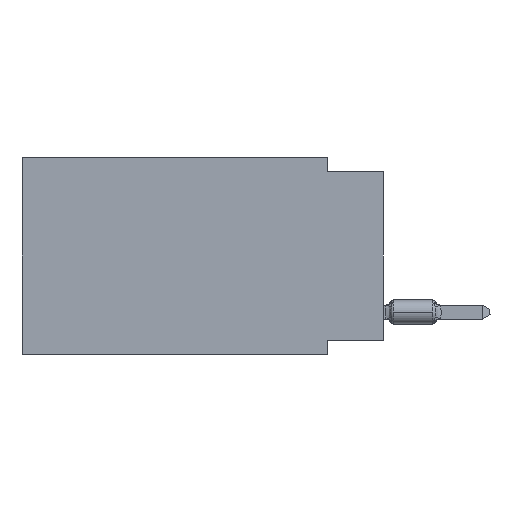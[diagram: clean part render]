
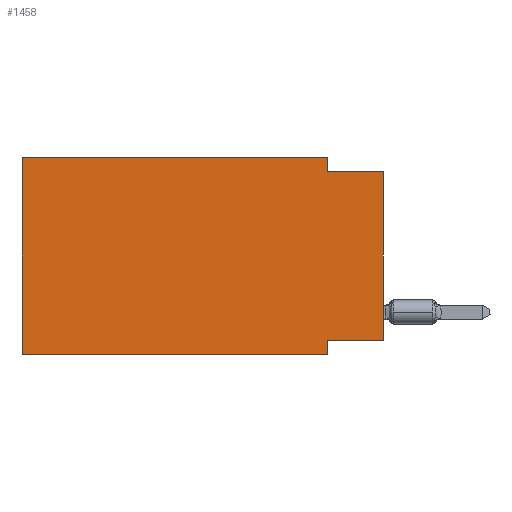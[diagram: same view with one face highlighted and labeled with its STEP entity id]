
A CAD part, left-side view. The second image highlights one B-rep face of the part: STEP entity #1458.
In plain terms, the highlighted planar face has unit normal (-1, 0, 0).
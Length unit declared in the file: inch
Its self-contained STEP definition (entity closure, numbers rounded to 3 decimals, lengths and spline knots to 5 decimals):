
#38 = VERTEX_POINT ( 'NONE', #5850 ) ;
#789 = DIRECTION ( 'NONE',  ( 1., 0., 0. ) ) ;
#1031 = LINE ( 'NONE', #18066, #4574 ) ;
#1359 = CARTESIAN_POINT ( 'NONE',  ( 0., 0., 0. ) ) ;
#1458 = ADVANCED_FACE ( 'NONE', ( #35137 ), #30677, .F. ) ;
#2916 = ORIENTED_EDGE ( 'NONE', *, *, #30691, .F. ) ;
#3138 = CARTESIAN_POINT ( 'NONE',  ( 0., 0.645, 0. ) ) ;
#4574 = VECTOR ( 'NONE', #35098, 39.37008 ) ;
#4625 = VERTEX_POINT ( 'NONE', #49537 ) ;
#5850 = CARTESIAN_POINT ( 'NONE',  ( 0., 0.1, 0. ) ) ;
#7056 = EDGE_CURVE ( 'NONE', #47800, #4625, #20248, .T. ) ;
#7983 = VECTOR ( 'NONE', #36603, 39.37008 ) ;
#9084 = CARTESIAN_POINT ( 'NONE',  ( 0., 0.1, -0.025 ) ) ;
#9440 = LINE ( 'NONE', #1359, #35969 ) ;
#10559 = DIRECTION ( 'NONE',  ( 0., 0., -1. ) ) ;
#11693 = DIRECTION ( 'NONE',  ( 0., 0., -1. ) ) ;
#12225 = EDGE_CURVE ( 'NONE', #38, #33472, #21179, .T. ) ;
#12871 = CARTESIAN_POINT ( 'NONE',  ( 0., 0., -0.025 ) ) ;
#13018 = CARTESIAN_POINT ( 'NONE',  ( 0., 0.645, -0.35 ) ) ;
#14031 = CARTESIAN_POINT ( 'NONE',  ( 0., 0.1, -0.325 ) ) ;
#14522 = CARTESIAN_POINT ( 'NONE',  ( 0., 0.645, 0. ) ) ;
#15605 = LINE ( 'NONE', #41816, #27776 ) ;
#15876 = ORIENTED_EDGE ( 'NONE', *, *, #7056, .T. ) ;
#16761 = CARTESIAN_POINT ( 'NONE',  ( 0., 0.645, 0. ) ) ;
#18066 = CARTESIAN_POINT ( 'NONE',  ( 0., 0., -0.325 ) ) ;
#20248 = LINE ( 'NONE', #37550, #31926 ) ;
#21179 = LINE ( 'NONE', #50003, #24462 ) ;
#22285 = DIRECTION ( 'NONE',  ( 0., 0., -1. ) ) ;
#24462 = VECTOR ( 'NONE', #11693, 39.37008 ) ;
#26155 = VECTOR ( 'NONE', #51140, 39.37008 ) ;
#26916 = EDGE_CURVE ( 'NONE', #40049, #4625, #27900, .T. ) ;
#27372 = ORIENTED_EDGE ( 'NONE', *, *, #12225, .F. ) ;
#27585 = CARTESIAN_POINT ( 'NONE',  ( 0., 0., -0.325 ) ) ;
#27670 = LINE ( 'NONE', #14522, #7983 ) ;
#27776 = VECTOR ( 'NONE', #32632, 39.37008 ) ;
#27900 = LINE ( 'NONE', #32349, #47503 ) ;
#30677 = PLANE ( 'NONE',  #54883 ) ;
#30691 = EDGE_CURVE ( 'NONE', #42112, #40049, #1031, .T. ) ;
#30851 = ORIENTED_EDGE ( 'NONE', *, *, #53261, .F. ) ;
#31926 = VECTOR ( 'NONE', #41482, 39.37008 ) ;
#32349 = CARTESIAN_POINT ( 'NONE',  ( 0., 0.1, -0.35 ) ) ;
#32453 = EDGE_CURVE ( 'NONE', #42112, #51260, #9440, .T. ) ;
#32632 = DIRECTION ( 'NONE',  ( 0., -1., 0. ) ) ;
#33078 = EDGE_CURVE ( 'NONE', #51153, #38, #46392, .T. ) ;
#33275 = ORIENTED_EDGE ( 'NONE', *, *, #26916, .F. ) ;
#33472 = VERTEX_POINT ( 'NONE', #9084 ) ;
#35098 = DIRECTION ( 'NONE',  ( 0., 1., 0. ) ) ;
#35137 = FACE_OUTER_BOUND ( 'NONE', #50706, .T. ) ;
#35418 = DIRECTION ( 'NONE',  ( 0., 0., 1. ) ) ;
#35969 = VECTOR ( 'NONE', #35418, 39.37008 ) ;
#36603 = DIRECTION ( 'NONE',  ( 0., 0., 1. ) ) ;
#37550 = CARTESIAN_POINT ( 'NONE',  ( 0., 0.645, -0.35 ) ) ;
#37971 = ORIENTED_EDGE ( 'NONE', *, *, #33078, .F. ) ;
#40049 = VERTEX_POINT ( 'NONE', #14031 ) ;
#40075 = ORIENTED_EDGE ( 'NONE', *, *, #51459, .F. ) ;
#41482 = DIRECTION ( 'NONE',  ( 0., -1., 0. ) ) ;
#41816 = CARTESIAN_POINT ( 'NONE',  ( 0., 0., -0.025 ) ) ;
#42112 = VERTEX_POINT ( 'NONE', #27585 ) ;
#44654 = ORIENTED_EDGE ( 'NONE', *, *, #32453, .T. ) ;
#46392 = LINE ( 'NONE', #16761, #26155 ) ;
#47503 = VECTOR ( 'NONE', #10559, 39.37008 ) ;
#47800 = VERTEX_POINT ( 'NONE', #13018 ) ;
#49537 = CARTESIAN_POINT ( 'NONE',  ( 0., 0.1, -0.35 ) ) ;
#50003 = CARTESIAN_POINT ( 'NONE',  ( 0., 0.1, 0. ) ) ;
#50706 = EDGE_LOOP ( 'NONE', ( #44654, #30851, #27372, #37971, #40075, #15876, #33275, #2916 ) ) ;
#51140 = DIRECTION ( 'NONE',  ( 0., -1., 0. ) ) ;
#51153 = VERTEX_POINT ( 'NONE', #3138 ) ;
#51260 = VERTEX_POINT ( 'NONE', #12871 ) ;
#51459 = EDGE_CURVE ( 'NONE', #47800, #51153, #27670, .T. ) ;
#52197 = CARTESIAN_POINT ( 'NONE',  ( 0., 0.645, 0. ) ) ;
#53261 = EDGE_CURVE ( 'NONE', #33472, #51260, #15605, .T. ) ;
#54883 = AXIS2_PLACEMENT_3D ( 'NONE', #52197, #789, #22285 ) ;
